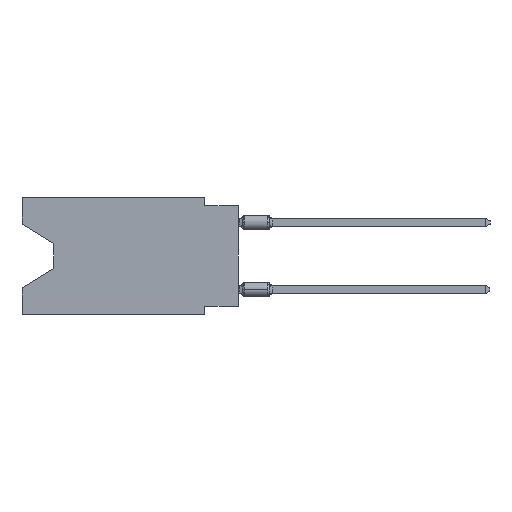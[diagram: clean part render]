
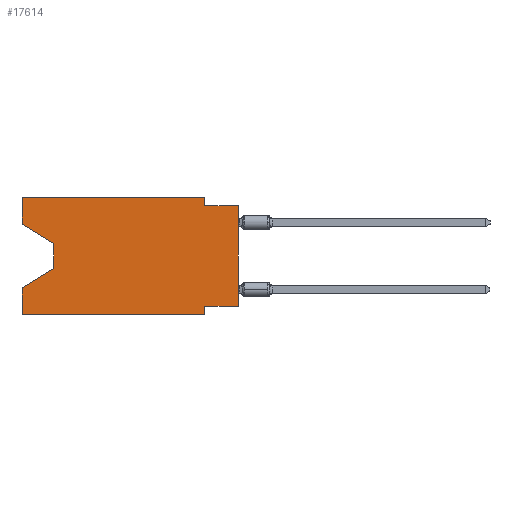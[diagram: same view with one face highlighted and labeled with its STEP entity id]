
A CAD part, left-side view. The second image highlights one B-rep face of the part: STEP entity #17614.
In plain terms, the highlighted planar face has unit normal (-1, 0, 0).
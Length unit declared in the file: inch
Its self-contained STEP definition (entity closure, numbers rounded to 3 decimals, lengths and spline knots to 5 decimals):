
#540 = VECTOR ( 'NONE', #15190, 39.37008 ) ;
#605 = VECTOR ( 'NONE', #1949, 39.37008 ) ;
#702 = EDGE_CURVE ( 'NONE', #18536, #16049, #2208, .T. ) ;
#774 = CARTESIAN_POINT ( 'NONE',  ( 0., 0., -0.025 ) ) ;
#811 = DIRECTION ( 'NONE',  ( 0., 0., -1. ) ) ;
#1224 = CARTESIAN_POINT ( 'NONE',  ( 0., 0.645, -0.08025 ) ) ;
#1336 = EDGE_LOOP ( 'NONE', ( #7615, #22180, #2424, #21403, #2056, #16165, #3258, #14154, #10162, #1921, #4941, #22209 ) ) ;
#1590 = DIRECTION ( 'NONE',  ( 0., 1., 0. ) ) ;
#1656 = CARTESIAN_POINT ( 'NONE',  ( 0., 0.1, 0. ) ) ;
#1711 = VERTEX_POINT ( 'NONE', #5870 ) ;
#1714 = DIRECTION ( 'NONE',  ( 0., 0.855, -0.519 ) ) ;
#1921 = ORIENTED_EDGE ( 'NONE', *, *, #12039, .F. ) ;
#1949 = DIRECTION ( 'NONE',  ( 0., 0., -1. ) ) ;
#2056 = ORIENTED_EDGE ( 'NONE', *, *, #11426, .T. ) ;
#2208 = LINE ( 'NONE', #17451, #22658 ) ;
#2323 = CARTESIAN_POINT ( 'NONE',  ( 0., 0.645, 0. ) ) ;
#2424 = ORIENTED_EDGE ( 'NONE', *, *, #15604, .T. ) ;
#2867 = LINE ( 'NONE', #1224, #14488 ) ;
#2923 = DIRECTION ( 'NONE',  ( 0., 0., 1. ) ) ;
#3172 = DIRECTION ( 'NONE',  ( 0., 0., -1. ) ) ;
#3258 = ORIENTED_EDGE ( 'NONE', *, *, #10757, .F. ) ;
#3444 = VERTEX_POINT ( 'NONE', #20927 ) ;
#3597 = CARTESIAN_POINT ( 'NONE',  ( 0., 0.55, -0.212 ) ) ;
#3862 = DIRECTION ( 'NONE',  ( 0., 0., -1. ) ) ;
#4155 = CARTESIAN_POINT ( 'NONE',  ( 0., 0.1, -0.025 ) ) ;
#4627 = CARTESIAN_POINT ( 'NONE',  ( 0., 0.645, -0.35 ) ) ;
#4694 = VECTOR ( 'NONE', #6759, 39.37008 ) ;
#4941 = ORIENTED_EDGE ( 'NONE', *, *, #15083, .F. ) ;
#5502 = LINE ( 'NONE', #3597, #9026 ) ;
#5661 = DIRECTION ( 'NONE',  ( 0., 0., 1. ) ) ;
#5760 = LINE ( 'NONE', #13361, #18123 ) ;
#5870 = CARTESIAN_POINT ( 'NONE',  ( 0., 0.55, -0.138 ) ) ;
#5908 = VERTEX_POINT ( 'NONE', #15298 ) ;
#6759 = DIRECTION ( 'NONE',  ( 0., -1., 0. ) ) ;
#6933 = EDGE_CURVE ( 'NONE', #5908, #1711, #2867, .T. ) ;
#6977 = CARTESIAN_POINT ( 'NONE',  ( 0., 0.1, -0.325 ) ) ;
#7489 = LINE ( 'NONE', #12972, #7842 ) ;
#7509 = CARTESIAN_POINT ( 'NONE',  ( 0., 0., -0.325 ) ) ;
#7615 = ORIENTED_EDGE ( 'NONE', *, *, #6933, .T. ) ;
#7770 = LINE ( 'NONE', #22747, #18206 ) ;
#7842 = VECTOR ( 'NONE', #1590, 39.37008 ) ;
#7978 = DIRECTION ( 'NONE',  ( 0., -1., 0. ) ) ;
#8212 = PLANE ( 'NONE',  #19026 ) ;
#8815 = EDGE_CURVE ( 'NONE', #23605, #16049, #21926, .T. ) ;
#9026 = VECTOR ( 'NONE', #1714, 39.37008 ) ;
#9489 = CARTESIAN_POINT ( 'NONE',  ( 0., 0.1, -0.35 ) ) ;
#9816 = EDGE_CURVE ( 'NONE', #13779, #13470, #24271, .T. ) ;
#10162 = ORIENTED_EDGE ( 'NONE', *, *, #702, .F. ) ;
#10491 = LINE ( 'NONE', #4627, #4694 ) ;
#10566 = CARTESIAN_POINT ( 'NONE',  ( 0., 0.55, -0.212 ) ) ;
#10757 = EDGE_CURVE ( 'NONE', #23605, #13779, #7489, .T. ) ;
#10915 = CARTESIAN_POINT ( 'NONE',  ( 0., 0.1, -0.35 ) ) ;
#11426 = EDGE_CURVE ( 'NONE', #15128, #13470, #10491, .T. ) ;
#12039 = EDGE_CURVE ( 'NONE', #19304, #18536, #5760, .T. ) ;
#12972 = CARTESIAN_POINT ( 'NONE',  ( 0., 0., -0.325 ) ) ;
#13361 = CARTESIAN_POINT ( 'NONE',  ( 0., 0.1, 0. ) ) ;
#13470 = VERTEX_POINT ( 'NONE', #9489 ) ;
#13579 = CARTESIAN_POINT ( 'NONE',  ( 0., 0.645, -0.35 ) ) ;
#13779 = VERTEX_POINT ( 'NONE', #6977 ) ;
#14049 = CARTESIAN_POINT ( 'NONE',  ( 0., 0., 0. ) ) ;
#14107 = LINE ( 'NONE', #21735, #21907 ) ;
#14154 = ORIENTED_EDGE ( 'NONE', *, *, #8815, .T. ) ;
#14236 = DIRECTION ( 'NONE',  ( 0., 0., 1. ) ) ;
#14344 = EDGE_CURVE ( 'NONE', #5908, #17160, #7770, .T. ) ;
#14488 = VECTOR ( 'NONE', #20102, 39.37008 ) ;
#15083 = EDGE_CURVE ( 'NONE', #17160, #19304, #19058, .T. ) ;
#15100 = EDGE_CURVE ( 'NONE', #1711, #20228, #17186, .T. ) ;
#15128 = VERTEX_POINT ( 'NONE', #13579 ) ;
#15190 = DIRECTION ( 'NONE',  ( 0., -1., 0. ) ) ;
#15298 = CARTESIAN_POINT ( 'NONE',  ( 0., 0.645, -0.08025 ) ) ;
#15604 = EDGE_CURVE ( 'NONE', #20228, #3444, #5502, .T. ) ;
#16049 = VERTEX_POINT ( 'NONE', #774 ) ;
#16165 = ORIENTED_EDGE ( 'NONE', *, *, #9816, .F. ) ;
#17160 = VERTEX_POINT ( 'NONE', #19583 ) ;
#17186 = LINE ( 'NONE', #20695, #605 ) ;
#17451 = CARTESIAN_POINT ( 'NONE',  ( 0., 0., -0.025 ) ) ;
#17613 = VECTOR ( 'NONE', #3172, 39.37008 ) ;
#17614 = ADVANCED_FACE ( 'NONE', ( #21821 ), #8212, .F. ) ;
#18123 = VECTOR ( 'NONE', #3862, 39.37008 ) ;
#18206 = VECTOR ( 'NONE', #5661, 39.37008 ) ;
#18536 = VERTEX_POINT ( 'NONE', #4155 ) ;
#18930 = CARTESIAN_POINT ( 'NONE',  ( 0., 0.645, 0. ) ) ;
#18998 = EDGE_CURVE ( 'NONE', #15128, #3444, #14107, .T. ) ;
#19026 = AXIS2_PLACEMENT_3D ( 'NONE', #2323, #19676, #811 ) ;
#19058 = LINE ( 'NONE', #18930, #540 ) ;
#19304 = VERTEX_POINT ( 'NONE', #1656 ) ;
#19583 = CARTESIAN_POINT ( 'NONE',  ( 0., 0.645, 0. ) ) ;
#19676 = DIRECTION ( 'NONE',  ( 1., 0., 0. ) ) ;
#20102 = DIRECTION ( 'NONE',  ( 0., -0.855, -0.519 ) ) ;
#20228 = VERTEX_POINT ( 'NONE', #10566 ) ;
#20695 = CARTESIAN_POINT ( 'NONE',  ( 0., 0.55, -0.138 ) ) ;
#20927 = CARTESIAN_POINT ( 'NONE',  ( 0., 0.645, -0.26975 ) ) ;
#21403 = ORIENTED_EDGE ( 'NONE', *, *, #18998, .F. ) ;
#21735 = CARTESIAN_POINT ( 'NONE',  ( 0., 0.645, 0. ) ) ;
#21821 = FACE_OUTER_BOUND ( 'NONE', #1336, .T. ) ;
#21907 = VECTOR ( 'NONE', #14236, 39.37008 ) ;
#21926 = LINE ( 'NONE', #14049, #22833 ) ;
#22180 = ORIENTED_EDGE ( 'NONE', *, *, #15100, .T. ) ;
#22209 = ORIENTED_EDGE ( 'NONE', *, *, #14344, .F. ) ;
#22658 = VECTOR ( 'NONE', #7978, 39.37008 ) ;
#22747 = CARTESIAN_POINT ( 'NONE',  ( 0., 0.645, 0. ) ) ;
#22833 = VECTOR ( 'NONE', #2923, 39.37008 ) ;
#23605 = VERTEX_POINT ( 'NONE', #7509 ) ;
#24271 = LINE ( 'NONE', #10915, #17613 ) ;
